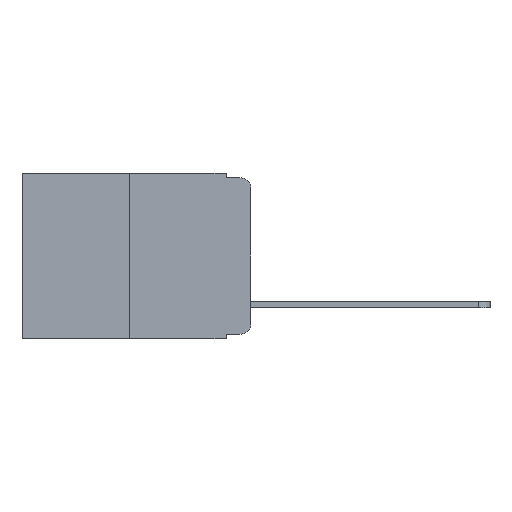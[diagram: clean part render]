
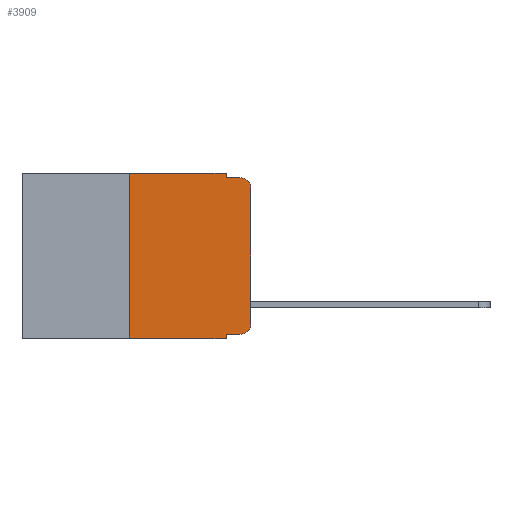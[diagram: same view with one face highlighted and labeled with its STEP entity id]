
A CAD part, left-side view. The second image highlights one B-rep face of the part: STEP entity #3909.
In plain terms, the highlighted planar face has unit normal (-1, 0, 0).
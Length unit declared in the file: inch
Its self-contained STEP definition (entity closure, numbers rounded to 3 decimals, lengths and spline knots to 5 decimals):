
#5 = ORIENTED_EDGE ( 'NONE', *, *, #7657, .T. ) ;
#104 = ORIENTED_EDGE ( 'NONE', *, *, #7636, .T. ) ;
#106 = CARTESIAN_POINT ( 'NONE',  ( 0., 0.02, -0.03 ) ) ;
#205 = ORIENTED_EDGE ( 'NONE', *, *, #7605, .F. ) ;
#275 = VERTEX_POINT ( 'NONE', #7228 ) ;
#489 = FACE_OUTER_BOUND ( 'NONE', #4413, .T. ) ;
#553 = CARTESIAN_POINT ( 'NONE',  ( 0., 0., 0. ) ) ;
#646 = DIRECTION ( 'NONE',  ( 0., 0., 1. ) ) ;
#697 = ORIENTED_EDGE ( 'NONE', *, *, #6589, .T. ) ;
#1101 = CARTESIAN_POINT ( 'NONE',  ( 0., 0.473, 0. ) ) ;
#1186 = LINE ( 'NONE', #553, #8790 ) ;
#1264 = AXIS2_PLACEMENT_3D ( 'NONE', #1101, #6433, #6429 ) ;
#1279 = EDGE_CURVE ( 'NONE', #3903, #8461, #11100, .T. ) ;
#1532 = ORIENTED_EDGE ( 'NONE', *, *, #7107, .F. ) ;
#1958 = CARTESIAN_POINT ( 'NONE',  ( 0., 0.02, -0.333 ) ) ;
#2389 = EDGE_CURVE ( 'NONE', #2892, #11075, #6178, .T. ) ;
#2892 = VERTEX_POINT ( 'NONE', #12265 ) ;
#2995 = CIRCLE ( 'NONE', #3305, 0.02 ) ;
#3179 = CARTESIAN_POINT ( 'NONE',  ( 0., 0.051, 0. ) ) ;
#3305 = AXIS2_PLACEMENT_3D ( 'NONE', #106, #11294, #6677 ) ;
#3399 = VERTEX_POINT ( 'NONE', #1958 ) ;
#3477 = VECTOR ( 'NONE', #3979, 39.37008 ) ;
#3702 = VECTOR ( 'NONE', #10419, 39.37008 ) ;
#3903 = VERTEX_POINT ( 'NONE', #4375 ) ;
#3909 = ADVANCED_FACE ( 'NONE', ( #489 ), #6476, .F. ) ;
#3979 = DIRECTION ( 'NONE',  ( 0., -1., 0. ) ) ;
#4075 = CIRCLE ( 'NONE', #4522, 0.02 ) ;
#4089 = VECTOR ( 'NONE', #11267, 39.37008 ) ;
#4375 = CARTESIAN_POINT ( 'NONE',  ( 0., 0.25, -0.343 ) ) ;
#4413 = EDGE_LOOP ( 'NONE', ( #697, #5204, #1532, #4924, #4891, #6241, #6105, #205, #104, #5 ) ) ;
#4522 = AXIS2_PLACEMENT_3D ( 'NONE', #10573, #10084, #9925 ) ;
#4534 = CARTESIAN_POINT ( 'NONE',  ( 0., 0.051, -0.01 ) ) ;
#4735 = LINE ( 'NONE', #6398, #6680 ) ;
#4888 = VERTEX_POINT ( 'NONE', #11637 ) ;
#4891 = ORIENTED_EDGE ( 'NONE', *, *, #2389, .F. ) ;
#4924 = ORIENTED_EDGE ( 'NONE', *, *, #7195, .F. ) ;
#5028 = VERTEX_POINT ( 'NONE', #12601 ) ;
#5118 = CARTESIAN_POINT ( 'NONE',  ( 0., 0.473, -0.343 ) ) ;
#5204 = ORIENTED_EDGE ( 'NONE', *, *, #6679, .T. ) ;
#5471 = DIRECTION ( 'NONE',  ( 0., -1., 0. ) ) ;
#5760 = VERTEX_POINT ( 'NONE', #4534 ) ;
#5813 = CARTESIAN_POINT ( 'NONE',  ( 0., 0.25, 0. ) ) ;
#6072 = VECTOR ( 'NONE', #9721, 39.37008 ) ;
#6105 = ORIENTED_EDGE ( 'NONE', *, *, #1279, .T. ) ;
#6178 = LINE ( 'NONE', #9037, #3477 ) ;
#6241 = ORIENTED_EDGE ( 'NONE', *, *, #7248, .F. ) ;
#6381 = DIRECTION ( 'NONE',  ( 0., 0., -1. ) ) ;
#6398 = CARTESIAN_POINT ( 'NONE',  ( 0., 0.051, -0.333 ) ) ;
#6429 = DIRECTION ( 'NONE',  ( 0., 0., -1. ) ) ;
#6433 = DIRECTION ( 'NONE',  ( 1., 0., 0. ) ) ;
#6476 = PLANE ( 'NONE',  #1264 ) ;
#6589 = EDGE_CURVE ( 'NONE', #275, #4888, #1186, .T. ) ;
#6677 = DIRECTION ( 'NONE',  ( 0., 0., -1. ) ) ;
#6679 = EDGE_CURVE ( 'NONE', #4888, #7886, #2995, .T. ) ;
#6680 = VECTOR ( 'NONE', #5471, 39.37008 ) ;
#7107 = EDGE_CURVE ( 'NONE', #5760, #7886, #11372, .T. ) ;
#7195 = EDGE_CURVE ( 'NONE', #11075, #5760, #8511, .T. ) ;
#7228 = CARTESIAN_POINT ( 'NONE',  ( 0., 0., -0.313 ) ) ;
#7248 = EDGE_CURVE ( 'NONE', #3903, #2892, #8255, .T. ) ;
#7276 = LINE ( 'NONE', #10457, #9309 ) ;
#7605 = EDGE_CURVE ( 'NONE', #5028, #8461, #7276, .T. ) ;
#7636 = EDGE_CURVE ( 'NONE', #5028, #3399, #4735, .T. ) ;
#7657 = EDGE_CURVE ( 'NONE', #3399, #275, #4075, .T. ) ;
#7738 = DIRECTION ( 'NONE',  ( 0., 0., 1. ) ) ;
#7886 = VERTEX_POINT ( 'NONE', #12620 ) ;
#8255 = LINE ( 'NONE', #5813, #12464 ) ;
#8461 = VERTEX_POINT ( 'NONE', #10007 ) ;
#8511 = LINE ( 'NONE', #11522, #6072 ) ;
#8790 = VECTOR ( 'NONE', #646, 39.37008 ) ;
#9037 = CARTESIAN_POINT ( 'NONE',  ( 0., 0.473, 0. ) ) ;
#9309 = VECTOR ( 'NONE', #6381, 39.37008 ) ;
#9721 = DIRECTION ( 'NONE',  ( 0., 0., -1. ) ) ;
#9925 = DIRECTION ( 'NONE',  ( 0., 0., -1. ) ) ;
#10007 = CARTESIAN_POINT ( 'NONE',  ( 0., 0.051, -0.343 ) ) ;
#10084 = DIRECTION ( 'NONE',  ( -1., 0., 0. ) ) ;
#10419 = DIRECTION ( 'NONE',  ( 0., -1., 0. ) ) ;
#10457 = CARTESIAN_POINT ( 'NONE',  ( 0., 0.051, 0. ) ) ;
#10573 = CARTESIAN_POINT ( 'NONE',  ( 0., 0.02, -0.313 ) ) ;
#10854 = CARTESIAN_POINT ( 'NONE',  ( 0., 0.051, -0.01 ) ) ;
#11075 = VERTEX_POINT ( 'NONE', #3179 ) ;
#11100 = LINE ( 'NONE', #5118, #3702 ) ;
#11267 = DIRECTION ( 'NONE',  ( 0., -1., 0. ) ) ;
#11294 = DIRECTION ( 'NONE',  ( -1., 0., 0. ) ) ;
#11372 = LINE ( 'NONE', #10854, #4089 ) ;
#11522 = CARTESIAN_POINT ( 'NONE',  ( 0., 0.051, 0. ) ) ;
#11637 = CARTESIAN_POINT ( 'NONE',  ( 0., 0., -0.03 ) ) ;
#12265 = CARTESIAN_POINT ( 'NONE',  ( 0., 0.25, 0. ) ) ;
#12464 = VECTOR ( 'NONE', #7738, 39.37008 ) ;
#12601 = CARTESIAN_POINT ( 'NONE',  ( 0., 0.051, -0.333 ) ) ;
#12620 = CARTESIAN_POINT ( 'NONE',  ( 0., 0.02, -0.01 ) ) ;
